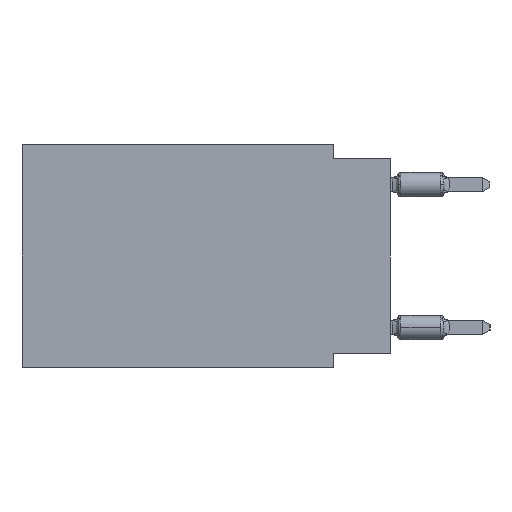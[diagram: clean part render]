
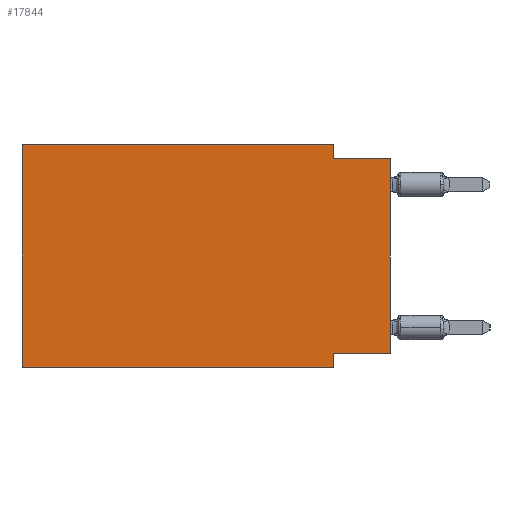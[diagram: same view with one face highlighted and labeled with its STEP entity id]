
A CAD part, left-side view. The second image highlights one B-rep face of the part: STEP entity #17844.
In plain terms, the highlighted planar face has unit normal (-1, 0, 0).
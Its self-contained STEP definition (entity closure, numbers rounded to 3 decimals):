
#23 = CARTESIAN_POINT ( 'NONE',  ( 0., 16.383, 0. ) ) ;
#108 = VERTEX_POINT ( 'NONE', #17946 ) ;
#682 = EDGE_CURVE ( 'NONE', #10056, #6913, #24664, .T. ) ;
#688 = EDGE_CURVE ( 'NONE', #4943, #8833, #20069, .T. ) ;
#759 = DIRECTION ( 'NONE',  ( 0., -1., 0. ) ) ;
#1419 = VERTEX_POINT ( 'NONE', #15435 ) ;
#1597 = VECTOR ( 'NONE', #759, 1000. ) ;
#1878 = ORIENTED_EDGE ( 'NONE', *, *, #19668, .F. ) ;
#2301 = LINE ( 'NONE', #24141, #5713 ) ;
#2348 = CARTESIAN_POINT ( 'NONE',  ( 0., 2.54, 0. ) ) ;
#2902 = CARTESIAN_POINT ( 'NONE',  ( 0., 16.383, 0. ) ) ;
#3495 = VECTOR ( 'NONE', #6488, 1000. ) ;
#3867 = CARTESIAN_POINT ( 'NONE',  ( 0., 16.383, -9.906 ) ) ;
#4753 = DIRECTION ( 'NONE',  ( 1., 0., 0. ) ) ;
#4943 = VERTEX_POINT ( 'NONE', #15821 ) ;
#4998 = DIRECTION ( 'NONE',  ( 0., 0., -1. ) ) ;
#5713 = VECTOR ( 'NONE', #14835, 1000. ) ;
#5776 = VECTOR ( 'NONE', #8744, 1000. ) ;
#6488 = DIRECTION ( 'NONE',  ( 0., 1., 0. ) ) ;
#6913 = VERTEX_POINT ( 'NONE', #8369 ) ;
#7066 = FACE_OUTER_BOUND ( 'NONE', #15346, .T. ) ;
#7250 = DIRECTION ( 'NONE',  ( 0., 0., -1. ) ) ;
#8369 = CARTESIAN_POINT ( 'NONE',  ( 0., 0., -0.635 ) ) ;
#8471 = LINE ( 'NONE', #3867, #5776 ) ;
#8744 = DIRECTION ( 'NONE',  ( 0., -1., 0. ) ) ;
#8833 = VERTEX_POINT ( 'NONE', #27671 ) ;
#9733 = CARTESIAN_POINT ( 'NONE',  ( 0., 0., -0.635 ) ) ;
#9769 = ORIENTED_EDGE ( 'NONE', *, *, #688, .F. ) ;
#10056 = VERTEX_POINT ( 'NONE', #17060 ) ;
#10265 = ORIENTED_EDGE ( 'NONE', *, *, #19825, .T. ) ;
#10676 = EDGE_CURVE ( 'NONE', #26824, #10056, #13862, .T. ) ;
#10798 = VECTOR ( 'NONE', #17265, 1000. ) ;
#10910 = ORIENTED_EDGE ( 'NONE', *, *, #20361, .T. ) ;
#10937 = VERTEX_POINT ( 'NONE', #18495 ) ;
#11087 = LINE ( 'NONE', #24152, #3495 ) ;
#12115 = CARTESIAN_POINT ( 'NONE',  ( 0., 2.54, 0. ) ) ;
#12292 = ORIENTED_EDGE ( 'NONE', *, *, #10676, .F. ) ;
#12449 = ORIENTED_EDGE ( 'NONE', *, *, #18780, .F. ) ;
#13007 = VECTOR ( 'NONE', #24516, 1000. ) ;
#13414 = PLANE ( 'NONE',  #23507 ) ;
#13862 = LINE ( 'NONE', #12115, #15941 ) ;
#14835 = DIRECTION ( 'NONE',  ( 0., 0., 1. ) ) ;
#15346 = EDGE_LOOP ( 'NONE', ( #10265, #16435, #12292, #1878, #12449, #10910, #9769, #26847 ) ) ;
#15435 = CARTESIAN_POINT ( 'NONE',  ( 0., 16.383, 0. ) ) ;
#15821 = CARTESIAN_POINT ( 'NONE',  ( 0., 2.54, -9.271 ) ) ;
#15941 = VECTOR ( 'NONE', #7250, 1000. ) ;
#16435 = ORIENTED_EDGE ( 'NONE', *, *, #682, .F. ) ;
#17060 = CARTESIAN_POINT ( 'NONE',  ( 0., 2.54, -0.635 ) ) ;
#17265 = DIRECTION ( 'NONE',  ( 0., 0., 1. ) ) ;
#17541 = DIRECTION ( 'NONE',  ( 0., 0., -1. ) ) ;
#17844 = ADVANCED_FACE ( 'NONE', ( #7066 ), #13414, .F. ) ;
#17946 = CARTESIAN_POINT ( 'NONE',  ( 0., 0., -9.271 ) ) ;
#18054 = CARTESIAN_POINT ( 'NONE',  ( 0., 2.54, -9.906 ) ) ;
#18476 = VECTOR ( 'NONE', #4998, 1000. ) ;
#18495 = CARTESIAN_POINT ( 'NONE',  ( 0., 16.383, -9.906 ) ) ;
#18780 = EDGE_CURVE ( 'NONE', #10937, #1419, #2301, .T. ) ;
#19119 = CARTESIAN_POINT ( 'NONE',  ( 0., 0., 0. ) ) ;
#19668 = EDGE_CURVE ( 'NONE', #1419, #26824, #22574, .T. ) ;
#19825 = EDGE_CURVE ( 'NONE', #108, #6913, #21274, .T. ) ;
#20069 = LINE ( 'NONE', #18054, #18476 ) ;
#20361 = EDGE_CURVE ( 'NONE', #10937, #8833, #8471, .T. ) ;
#21274 = LINE ( 'NONE', #19119, #10798 ) ;
#22574 = LINE ( 'NONE', #2902, #1597 ) ;
#23507 = AXIS2_PLACEMENT_3D ( 'NONE', #23, #4753, #17541 ) ;
#24141 = CARTESIAN_POINT ( 'NONE',  ( 0., 16.383, 0. ) ) ;
#24152 = CARTESIAN_POINT ( 'NONE',  ( 0., 0., -9.271 ) ) ;
#24516 = DIRECTION ( 'NONE',  ( 0., -1., 0. ) ) ;
#24664 = LINE ( 'NONE', #9733, #13007 ) ;
#26824 = VERTEX_POINT ( 'NONE', #2348 ) ;
#26847 = ORIENTED_EDGE ( 'NONE', *, *, #27163, .F. ) ;
#27163 = EDGE_CURVE ( 'NONE', #108, #4943, #11087, .T. ) ;
#27671 = CARTESIAN_POINT ( 'NONE',  ( 0., 2.54, -9.906 ) ) ;
